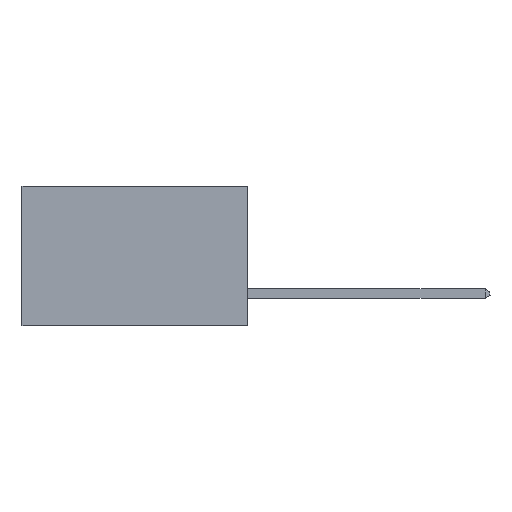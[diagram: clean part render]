
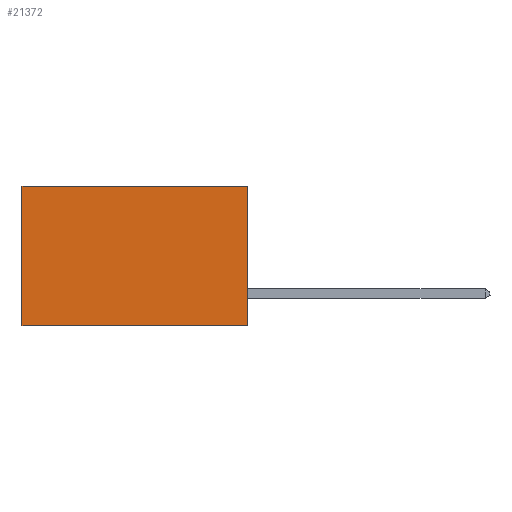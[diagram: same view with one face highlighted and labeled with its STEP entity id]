
A CAD part, left-side view. The second image highlights one B-rep face of the part: STEP entity #21372.
In plain terms, the highlighted planar face has unit normal (-1, 0, 0).
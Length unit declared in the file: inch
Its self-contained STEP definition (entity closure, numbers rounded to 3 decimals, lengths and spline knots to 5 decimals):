
#190 = VECTOR ( 'NONE', #24155, 39.37008 ) ;
#509 = CARTESIAN_POINT ( 'NONE',  ( 0.298, 0., -0.37 ) ) ;
#1085 = CARTESIAN_POINT ( 'NONE',  ( 0.298, 0., -0.37 ) ) ;
#1179 = ORIENTED_EDGE ( 'NONE', *, *, #25072, .F. ) ;
#1517 = PLANE ( 'NONE',  #10555 ) ;
#1538 = LINE ( 'NONE', #11057, #25233 ) ;
#2896 = FACE_OUTER_BOUND ( 'NONE', #8805, .T. ) ;
#3182 = CARTESIAN_POINT ( 'NONE',  ( 0.298, 0., 0. ) ) ;
#3547 = DIRECTION ( 'NONE',  ( 0., 1., 0. ) ) ;
#5209 = LINE ( 'NONE', #8900, #25326 ) ;
#6095 = CARTESIAN_POINT ( 'NONE',  ( 0.298, 0., 0. ) ) ;
#8103 = VERTEX_POINT ( 'NONE', #16020 ) ;
#8805 = EDGE_LOOP ( 'NONE', ( #22345, #23333, #1179, #22934 ) ) ;
#8900 = CARTESIAN_POINT ( 'NONE',  ( 0.298, 0., 0. ) ) ;
#10278 = VERTEX_POINT ( 'NONE', #29081 ) ;
#10555 = AXIS2_PLACEMENT_3D ( 'NONE', #6095, #22461, #26916 ) ;
#11057 = CARTESIAN_POINT ( 'NONE',  ( 0.298, 0.6, 0. ) ) ;
#14557 = LINE ( 'NONE', #14568, #26432 ) ;
#14568 = CARTESIAN_POINT ( 'NONE',  ( 0.298, 0., 0. ) ) ;
#16020 = CARTESIAN_POINT ( 'NONE',  ( 0.298, 0.6, 0. ) ) ;
#16022 = DIRECTION ( 'NONE',  ( 0., 0., -1. ) ) ;
#20163 = EDGE_CURVE ( 'NONE', #27311, #10278, #22782, .T. ) ;
#20834 = EDGE_CURVE ( 'NONE', #8103, #10278, #1538, .T. ) ;
#21372 = ADVANCED_FACE ( 'NONE', ( #2896 ), #1517, .F. ) ;
#21808 = VERTEX_POINT ( 'NONE', #3182 ) ;
#22345 = ORIENTED_EDGE ( 'NONE', *, *, #20834, .T. ) ;
#22461 = DIRECTION ( 'NONE',  ( 1., 0., 0. ) ) ;
#22782 = LINE ( 'NONE', #1085, #190 ) ;
#22934 = ORIENTED_EDGE ( 'NONE', *, *, #24842, .T. ) ;
#23333 = ORIENTED_EDGE ( 'NONE', *, *, #20163, .F. ) ;
#24155 = DIRECTION ( 'NONE',  ( 0., 1., 0. ) ) ;
#24842 = EDGE_CURVE ( 'NONE', #21808, #8103, #14557, .T. ) ;
#25072 = EDGE_CURVE ( 'NONE', #21808, #27311, #5209, .T. ) ;
#25233 = VECTOR ( 'NONE', #29631, 39.37008 ) ;
#25326 = VECTOR ( 'NONE', #16022, 39.37008 ) ;
#26432 = VECTOR ( 'NONE', #3547, 39.37008 ) ;
#26916 = DIRECTION ( 'NONE',  ( 0., 0., -1. ) ) ;
#27311 = VERTEX_POINT ( 'NONE', #509 ) ;
#29081 = CARTESIAN_POINT ( 'NONE',  ( 0.298, 0.6, -0.37 ) ) ;
#29631 = DIRECTION ( 'NONE',  ( 0., 0., -1. ) ) ;
